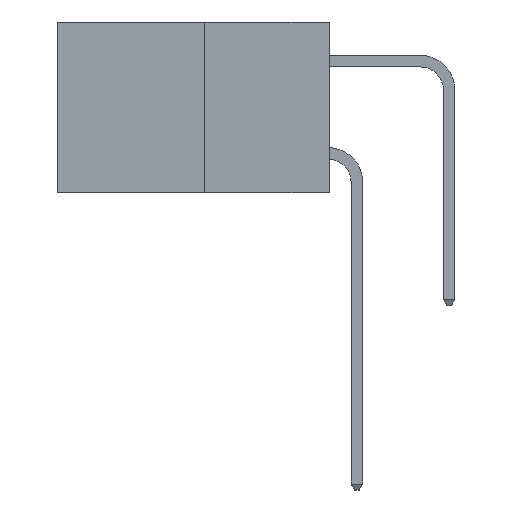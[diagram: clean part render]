
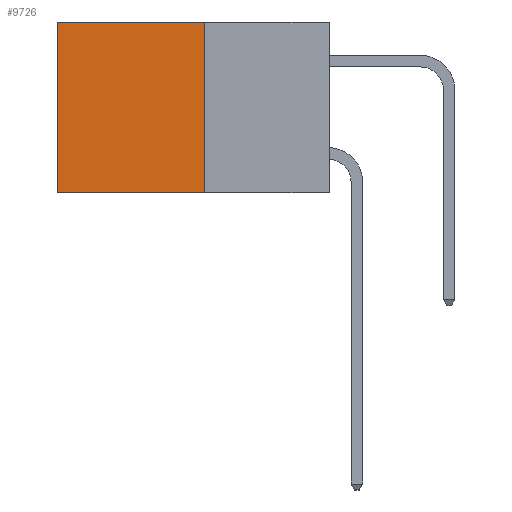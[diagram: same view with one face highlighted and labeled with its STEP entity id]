
A CAD part, left-side view. The second image highlights one B-rep face of the part: STEP entity #9726.
In plain terms, the highlighted planar face has unit normal (-1, 0, 0).
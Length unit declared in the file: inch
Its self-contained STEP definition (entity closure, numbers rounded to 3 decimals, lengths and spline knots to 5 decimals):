
#292 = CARTESIAN_POINT ( 'NONE',  ( 0.277, 0.27, -0.37 ) ) ;
#335 = DIRECTION ( 'NONE',  ( 0., 1., 0. ) ) ;
#684 = ORIENTED_EDGE ( 'NONE', *, *, #9212, .T. ) ;
#780 = CARTESIAN_POINT ( 'NONE',  ( 0.277, 0.59, -0.37 ) ) ;
#849 = DIRECTION ( 'NONE',  ( 0., 0., -1. ) ) ;
#932 = VERTEX_POINT ( 'NONE', #7563 ) ;
#1620 = VECTOR ( 'NONE', #6235, 39.37008 ) ;
#2472 = CARTESIAN_POINT ( 'NONE',  ( 0.277, 0.27, 0. ) ) ;
#2795 = VECTOR ( 'NONE', #849, 39.37008 ) ;
#2957 = LINE ( 'NONE', #292, #3243 ) ;
#3243 = VECTOR ( 'NONE', #335, 39.37008 ) ;
#3452 = EDGE_CURVE ( 'NONE', #5288, #8573, #2957, .T. ) ;
#3651 = EDGE_LOOP ( 'NONE', ( #684, #10094, #5795, #8133 ) ) ;
#4414 = VERTEX_POINT ( 'NONE', #9559 ) ;
#4802 = DIRECTION ( 'NONE',  ( 0., 0., -1. ) ) ;
#5288 = VERTEX_POINT ( 'NONE', #5503 ) ;
#5503 = CARTESIAN_POINT ( 'NONE',  ( 0.277, 0.27, -0.37 ) ) ;
#5795 = ORIENTED_EDGE ( 'NONE', *, *, #8610, .F. ) ;
#6049 = DIRECTION ( 'NONE',  ( 0., 1., 0. ) ) ;
#6235 = DIRECTION ( 'NONE',  ( 0., 0., -1. ) ) ;
#6268 = EDGE_CURVE ( 'NONE', #932, #4414, #9803, .T. ) ;
#7443 = PLANE ( 'NONE',  #9145 ) ;
#7551 = VECTOR ( 'NONE', #6049, 39.37008 ) ;
#7563 = CARTESIAN_POINT ( 'NONE',  ( 0.277, 0.27, 0. ) ) ;
#8133 = ORIENTED_EDGE ( 'NONE', *, *, #6268, .T. ) ;
#8573 = VERTEX_POINT ( 'NONE', #780 ) ;
#8610 = EDGE_CURVE ( 'NONE', #932, #5288, #10891, .T. ) ;
#8849 = CARTESIAN_POINT ( 'NONE',  ( 0.277, 0.27, -0.37 ) ) ;
#9145 = AXIS2_PLACEMENT_3D ( 'NONE', #9157, #9983, #4802 ) ;
#9157 = CARTESIAN_POINT ( 'NONE',  ( 0.277, 0.27, -0.37 ) ) ;
#9212 = EDGE_CURVE ( 'NONE', #4414, #8573, #9498, .T. ) ;
#9498 = LINE ( 'NONE', #11302, #2795 ) ;
#9559 = CARTESIAN_POINT ( 'NONE',  ( 0.277, 0.59, 0. ) ) ;
#9726 = ADVANCED_FACE ( 'NONE', ( #10885 ), #7443, .F. ) ;
#9803 = LINE ( 'NONE', #2472, #7551 ) ;
#9983 = DIRECTION ( 'NONE',  ( 1., 0., 0. ) ) ;
#10094 = ORIENTED_EDGE ( 'NONE', *, *, #3452, .F. ) ;
#10885 = FACE_OUTER_BOUND ( 'NONE', #3651, .T. ) ;
#10891 = LINE ( 'NONE', #8849, #1620 ) ;
#11302 = CARTESIAN_POINT ( 'NONE',  ( 0.277, 0.59, -0.37 ) ) ;
